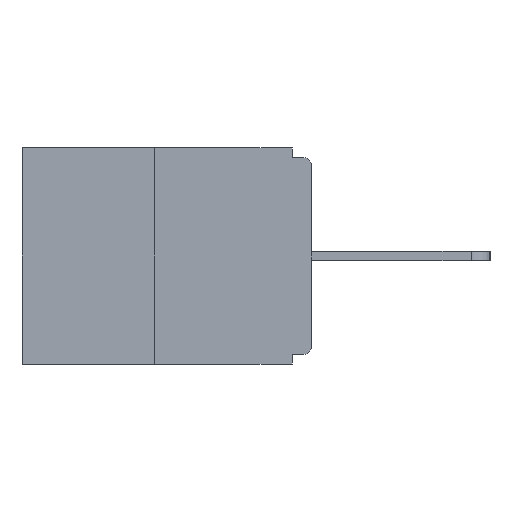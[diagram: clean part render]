
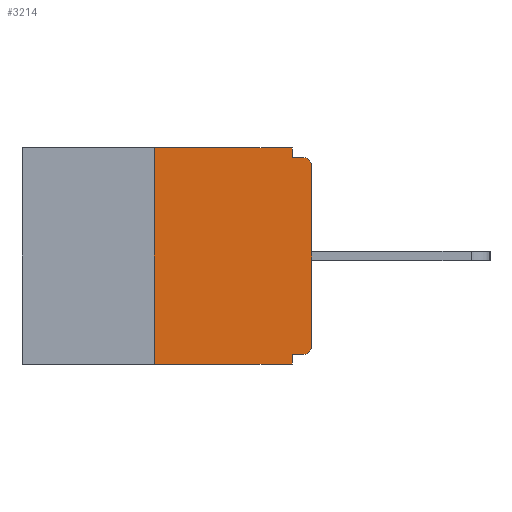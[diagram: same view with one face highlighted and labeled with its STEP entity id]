
A CAD part, left-side view. The second image highlights one B-rep face of the part: STEP entity #3214.
In plain terms, the highlighted planar face has unit normal (-1, 0, 0).
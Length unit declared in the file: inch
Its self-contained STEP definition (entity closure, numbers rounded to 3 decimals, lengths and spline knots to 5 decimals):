
#64 = CARTESIAN_POINT ( 'NONE',  ( 0., 0.25, 0. ) ) ;
#182 = LINE ( 'NONE', #13640, #14703 ) ;
#423 = EDGE_CURVE ( 'NONE', #14726, #1565, #11635, .T. ) ;
#733 = VECTOR ( 'NONE', #7418, 39.37008 ) ;
#799 = ORIENTED_EDGE ( 'NONE', *, *, #13147, .F. ) ;
#1078 = DIRECTION ( 'NONE',  ( 0., 0., -1. ) ) ;
#1090 = DIRECTION ( 'NONE',  ( 0., 1., 0. ) ) ;
#1260 = ORIENTED_EDGE ( 'NONE', *, *, #6522, .T. ) ;
#1336 = CARTESIAN_POINT ( 'NONE',  ( 0., 0.031, -0.343 ) ) ;
#1565 = VERTEX_POINT ( 'NONE', #11207 ) ;
#1690 = CARTESIAN_POINT ( 'NONE',  ( 0., 0., -0.328 ) ) ;
#1846 = VECTOR ( 'NONE', #1090, 39.37008 ) ;
#1857 = AXIS2_PLACEMENT_3D ( 'NONE', #8713, #9959, #9913 ) ;
#1961 = CARTESIAN_POINT ( 'NONE',  ( 0., 0.25, 0. ) ) ;
#2332 = LINE ( 'NONE', #1690, #1846 ) ;
#2608 = VERTEX_POINT ( 'NONE', #16402 ) ;
#2630 = CARTESIAN_POINT ( 'NONE',  ( 0., 0., 0. ) ) ;
#3214 = ADVANCED_FACE ( 'NONE', ( #15404 ), #8736, .F. ) ;
#3576 = ORIENTED_EDGE ( 'NONE', *, *, #11356, .F. ) ;
#4001 = ORIENTED_EDGE ( 'NONE', *, *, #423, .F. ) ;
#4038 = VERTEX_POINT ( 'NONE', #4175 ) ;
#4055 = VERTEX_POINT ( 'NONE', #4596 ) ;
#4056 = DIRECTION ( 'NONE',  ( 0., 0., 1. ) ) ;
#4065 = CARTESIAN_POINT ( 'NONE',  ( 0., 0., -0.03 ) ) ;
#4098 = VERTEX_POINT ( 'NONE', #12887 ) ;
#4175 = CARTESIAN_POINT ( 'NONE',  ( 0., 0.031, -0.328 ) ) ;
#4596 = CARTESIAN_POINT ( 'NONE',  ( 0., 0.015, -0.328 ) ) ;
#4774 = VECTOR ( 'NONE', #6711, 39.37008 ) ;
#5102 = CARTESIAN_POINT ( 'NONE',  ( 0., 0.015, -0.03 ) ) ;
#5128 = ORIENTED_EDGE ( 'NONE', *, *, #14341, .T. ) ;
#5161 = EDGE_CURVE ( 'NONE', #8547, #13158, #182, .T. ) ;
#5270 = EDGE_CURVE ( 'NONE', #4055, #4038, #2332, .T. ) ;
#5491 = AXIS2_PLACEMENT_3D ( 'NONE', #5102, #14732, #6533 ) ;
#5593 = CIRCLE ( 'NONE', #6306, 0.015 ) ;
#6027 = DIRECTION ( 'NONE',  ( -1., 0., 0. ) ) ;
#6306 = AXIS2_PLACEMENT_3D ( 'NONE', #14266, #6027, #15619 ) ;
#6437 = CIRCLE ( 'NONE', #5491, 0.015 ) ;
#6522 = EDGE_CURVE ( 'NONE', #4098, #2608, #15754, .T. ) ;
#6533 = DIRECTION ( 'NONE',  ( 0., 0., -1. ) ) ;
#6648 = EDGE_CURVE ( 'NONE', #4038, #2608, #16766, .T. ) ;
#6711 = DIRECTION ( 'NONE',  ( 0., -1., 0. ) ) ;
#6887 = VECTOR ( 'NONE', #4056, 39.37008 ) ;
#7017 = VERTEX_POINT ( 'NONE', #14032 ) ;
#7229 = CARTESIAN_POINT ( 'NONE',  ( 0., 0.46, -0.343 ) ) ;
#7299 = LINE ( 'NONE', #2630, #6887 ) ;
#7418 = DIRECTION ( 'NONE',  ( 0., 0., -1. ) ) ;
#7539 = LINE ( 'NONE', #1961, #10765 ) ;
#7553 = VECTOR ( 'NONE', #9313, 39.37008 ) ;
#8547 = VERTEX_POINT ( 'NONE', #11303 ) ;
#8713 = CARTESIAN_POINT ( 'NONE',  ( 0., 0.46, 0. ) ) ;
#8736 = PLANE ( 'NONE',  #1857 ) ;
#8796 = ORIENTED_EDGE ( 'NONE', *, *, #6648, .F. ) ;
#8873 = EDGE_LOOP ( 'NONE', ( #4001, #799, #1260, #8796, #11380, #9624, #10936, #5128, #10544, #3576 ) ) ;
#9313 = DIRECTION ( 'NONE',  ( 0., -1., 0. ) ) ;
#9624 = ORIENTED_EDGE ( 'NONE', *, *, #13027, .T. ) ;
#9913 = DIRECTION ( 'NONE',  ( 0., 0., -1. ) ) ;
#9959 = DIRECTION ( 'NONE',  ( 1., 0., 0. ) ) ;
#10418 = DIRECTION ( 'NONE',  ( 0., 0., 1. ) ) ;
#10544 = ORIENTED_EDGE ( 'NONE', *, *, #5161, .F. ) ;
#10607 = CARTESIAN_POINT ( 'NONE',  ( 0., 0.46, 0. ) ) ;
#10765 = VECTOR ( 'NONE', #10418, 39.37008 ) ;
#10936 = ORIENTED_EDGE ( 'NONE', *, *, #13854, .T. ) ;
#11207 = CARTESIAN_POINT ( 'NONE',  ( 0., 0.031, 0. ) ) ;
#11303 = CARTESIAN_POINT ( 'NONE',  ( 0., 0.031, -0.015 ) ) ;
#11356 = EDGE_CURVE ( 'NONE', #1565, #8547, #14743, .T. ) ;
#11380 = ORIENTED_EDGE ( 'NONE', *, *, #5270, .F. ) ;
#11635 = LINE ( 'NONE', #10607, #7553 ) ;
#11790 = CARTESIAN_POINT ( 'NONE',  ( 0., 0.015, -0.015 ) ) ;
#12887 = CARTESIAN_POINT ( 'NONE',  ( 0., 0.25, -0.343 ) ) ;
#13027 = EDGE_CURVE ( 'NONE', #4055, #7017, #5593, .T. ) ;
#13147 = EDGE_CURVE ( 'NONE', #4098, #14726, #7539, .T. ) ;
#13158 = VERTEX_POINT ( 'NONE', #11790 ) ;
#13640 = CARTESIAN_POINT ( 'NONE',  ( 0., 0., -0.015 ) ) ;
#13854 = EDGE_CURVE ( 'NONE', #7017, #16692, #7299, .T. ) ;
#14014 = DIRECTION ( 'NONE',  ( 0., -1., 0. ) ) ;
#14032 = CARTESIAN_POINT ( 'NONE',  ( 0., 0., -0.313 ) ) ;
#14266 = CARTESIAN_POINT ( 'NONE',  ( 0., 0.015, -0.313 ) ) ;
#14324 = CARTESIAN_POINT ( 'NONE',  ( 0., 0.031, 0. ) ) ;
#14341 = EDGE_CURVE ( 'NONE', #16692, #13158, #6437, .T. ) ;
#14703 = VECTOR ( 'NONE', #14014, 39.37008 ) ;
#14726 = VERTEX_POINT ( 'NONE', #64 ) ;
#14732 = DIRECTION ( 'NONE',  ( -1., 0., 0. ) ) ;
#14743 = LINE ( 'NONE', #14324, #733 ) ;
#15404 = FACE_OUTER_BOUND ( 'NONE', #8873, .T. ) ;
#15619 = DIRECTION ( 'NONE',  ( 0., 0., -1. ) ) ;
#15754 = LINE ( 'NONE', #7229, #4774 ) ;
#16402 = CARTESIAN_POINT ( 'NONE',  ( 0., 0.031, -0.343 ) ) ;
#16692 = VERTEX_POINT ( 'NONE', #4065 ) ;
#16766 = LINE ( 'NONE', #1336, #17177 ) ;
#17177 = VECTOR ( 'NONE', #1078, 39.37008 ) ;
